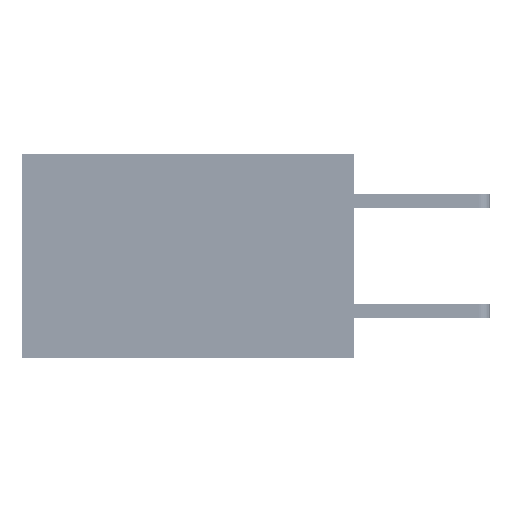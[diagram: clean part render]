
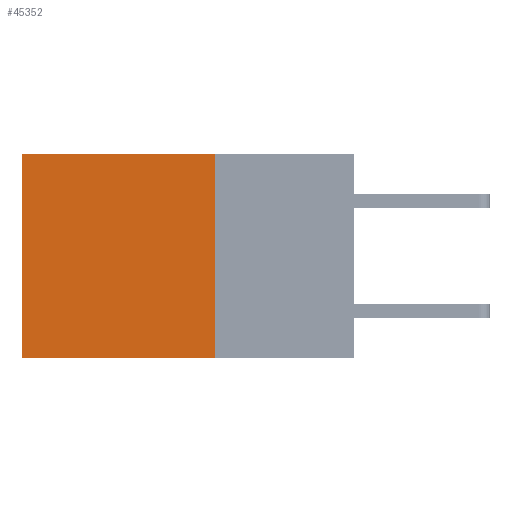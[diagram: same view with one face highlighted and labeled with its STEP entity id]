
A CAD part, left-side view. The second image highlights one B-rep face of the part: STEP entity #45352.
In plain terms, the highlighted planar face has unit normal (-1, 0, 0).
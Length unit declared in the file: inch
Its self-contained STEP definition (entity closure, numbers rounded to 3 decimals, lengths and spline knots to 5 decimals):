
#102 = VERTEX_POINT ( 'NONE', #9666 ) ;
#1303 = CARTESIAN_POINT ( 'NONE',  ( 0.2875, 0.25, -0.37 ) ) ;
#4993 = ORIENTED_EDGE ( 'NONE', *, *, #45945, .F. ) ;
#5435 = VECTOR ( 'NONE', #40126, 39.37008 ) ;
#7793 = VECTOR ( 'NONE', #31633, 39.37008 ) ;
#8201 = CARTESIAN_POINT ( 'NONE',  ( 0.2875, 0.6, -0.37 ) ) ;
#8243 = ORIENTED_EDGE ( 'NONE', *, *, #13411, .F. ) ;
#9666 = CARTESIAN_POINT ( 'NONE',  ( 0.2875, 0.6, 0. ) ) ;
#13411 = EDGE_CURVE ( 'NONE', #28879, #29047, #39425, .T. ) ;
#13542 = DIRECTION ( 'NONE',  ( 0., 1., 0. ) ) ;
#18095 = LINE ( 'NONE', #44211, #20007 ) ;
#20007 = VECTOR ( 'NONE', #43747, 39.37008 ) ;
#21814 = ORIENTED_EDGE ( 'NONE', *, *, #31857, .T. ) ;
#23162 = DIRECTION ( 'NONE',  ( 0., 0., -1. ) ) ;
#25320 = EDGE_LOOP ( 'NONE', ( #36364, #4993, #8243, #21814 ) ) ;
#28879 = VERTEX_POINT ( 'NONE', #30571 ) ;
#29047 = VERTEX_POINT ( 'NONE', #45935 ) ;
#30484 = CARTESIAN_POINT ( 'NONE',  ( 0.2875, 0.25, 0. ) ) ;
#30571 = CARTESIAN_POINT ( 'NONE',  ( 0.2875, 0.25, 0. ) ) ;
#31633 = DIRECTION ( 'NONE',  ( 0., 1., 0. ) ) ;
#31857 = EDGE_CURVE ( 'NONE', #28879, #102, #35783, .T. ) ;
#32120 = CARTESIAN_POINT ( 'NONE',  ( 0.2875, 0.25, 0. ) ) ;
#32815 = CARTESIAN_POINT ( 'NONE',  ( 0.2875, 0.25, 0. ) ) ;
#32904 = VERTEX_POINT ( 'NONE', #8201 ) ;
#34923 = VECTOR ( 'NONE', #13542, 39.37008 ) ;
#35783 = LINE ( 'NONE', #32120, #34923 ) ;
#36364 = ORIENTED_EDGE ( 'NONE', *, *, #41441, .T. ) ;
#38286 = DIRECTION ( 'NONE',  ( 1., 0., 0. ) ) ;
#38521 = PLANE ( 'NONE',  #45213 ) ;
#39425 = LINE ( 'NONE', #32815, #5435 ) ;
#40126 = DIRECTION ( 'NONE',  ( 0., 0., -1. ) ) ;
#41441 = EDGE_CURVE ( 'NONE', #102, #32904, #18095, .T. ) ;
#41703 = FACE_OUTER_BOUND ( 'NONE', #25320, .T. ) ;
#42362 = LINE ( 'NONE', #1303, #7793 ) ;
#43747 = DIRECTION ( 'NONE',  ( 0., 0., -1. ) ) ;
#44211 = CARTESIAN_POINT ( 'NONE',  ( 0.2875, 0.6, 0. ) ) ;
#45213 = AXIS2_PLACEMENT_3D ( 'NONE', #30484, #38286, #23162 ) ;
#45352 = ADVANCED_FACE ( 'NONE', ( #41703 ), #38521, .F. ) ;
#45935 = CARTESIAN_POINT ( 'NONE',  ( 0.2875, 0.25, -0.37 ) ) ;
#45945 = EDGE_CURVE ( 'NONE', #29047, #32904, #42362, .T. ) ;
